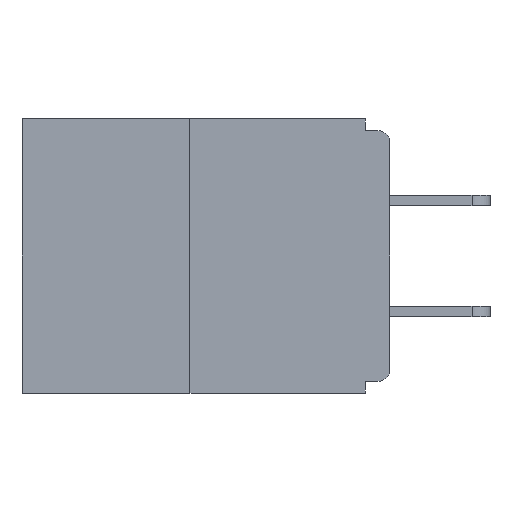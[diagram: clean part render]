
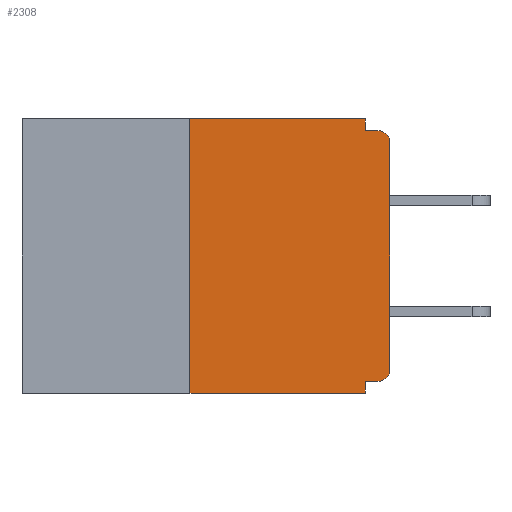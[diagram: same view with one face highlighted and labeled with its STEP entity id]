
A CAD part, left-side view. The second image highlights one B-rep face of the part: STEP entity #2308.
In plain terms, the highlighted planar face has unit normal (-1, 0, 0).
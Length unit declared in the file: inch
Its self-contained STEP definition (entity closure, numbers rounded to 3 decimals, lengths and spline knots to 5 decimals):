
#131 = CARTESIAN_POINT ( 'NONE',  ( 0., 0.25, -0.343 ) ) ;
#202 = CARTESIAN_POINT ( 'NONE',  ( 0., 0.46, 0. ) ) ;
#671 = DIRECTION ( 'NONE',  ( -1., 0., 0. ) ) ;
#1370 = VERTEX_POINT ( 'NONE', #13479 ) ;
#1559 = LINE ( 'NONE', #3961, #16559 ) ;
#1993 = DIRECTION ( 'NONE',  ( 0., 0., -1. ) ) ;
#2171 = DIRECTION ( 'NONE',  ( 0., -1., 0. ) ) ;
#2308 = ADVANCED_FACE ( 'NONE', ( #8596 ), #10376, .F. ) ;
#2383 = CARTESIAN_POINT ( 'NONE',  ( 0., 0.46, 0. ) ) ;
#2576 = VECTOR ( 'NONE', #9183, 39.37008 ) ;
#2650 = VERTEX_POINT ( 'NONE', #9824 ) ;
#3369 = EDGE_CURVE ( 'NONE', #5888, #11974, #8760, .T. ) ;
#3402 = CARTESIAN_POINT ( 'NONE',  ( 0., 0.25, 0. ) ) ;
#3457 = DIRECTION ( 'NONE',  ( -1., 0., 0. ) ) ;
#3500 = CARTESIAN_POINT ( 'NONE',  ( 0., 0.25, 0. ) ) ;
#3734 = VERTEX_POINT ( 'NONE', #15342 ) ;
#3848 = CARTESIAN_POINT ( 'NONE',  ( 0., 0., -0.03 ) ) ;
#3932 = EDGE_CURVE ( 'NONE', #2650, #1370, #5480, .T. ) ;
#3961 = CARTESIAN_POINT ( 'NONE',  ( 0., 0.46, -0.343 ) ) ;
#4158 = VECTOR ( 'NONE', #11463, 39.37008 ) ;
#4496 = VERTEX_POINT ( 'NONE', #15976 ) ;
#4717 = EDGE_CURVE ( 'NONE', #5970, #9330, #13332, .T. ) ;
#4718 = EDGE_CURVE ( 'NONE', #13329, #4496, #1559, .T. ) ;
#5480 = LINE ( 'NONE', #13097, #6284 ) ;
#5781 = AXIS2_PLACEMENT_3D ( 'NONE', #202, #12934, #7872 ) ;
#5888 = VERTEX_POINT ( 'NONE', #15579 ) ;
#5970 = VERTEX_POINT ( 'NONE', #11804 ) ;
#6000 = AXIS2_PLACEMENT_3D ( 'NONE', #8614, #671, #7072 ) ;
#6284 = VECTOR ( 'NONE', #15729, 39.37008 ) ;
#6303 = VECTOR ( 'NONE', #2171, 39.37008 ) ;
#6318 = AXIS2_PLACEMENT_3D ( 'NONE', #9764, #3457, #13645 ) ;
#6791 = DIRECTION ( 'NONE',  ( 0., 0., 1. ) ) ;
#7072 = DIRECTION ( 'NONE',  ( 0., 0., -1. ) ) ;
#7277 = CARTESIAN_POINT ( 'NONE',  ( 0., 0.031, 0. ) ) ;
#7509 = ORIENTED_EDGE ( 'NONE', *, *, #15427, .T. ) ;
#7675 = EDGE_LOOP ( 'NONE', ( #12702, #15462, #13352, #12269, #12485, #9810, #16734, #7509, #9203, #15698 ) ) ;
#7757 = LINE ( 'NONE', #3500, #10358 ) ;
#7872 = DIRECTION ( 'NONE',  ( 0., 0., -1. ) ) ;
#7903 = DIRECTION ( 'NONE',  ( 0., -1., 0. ) ) ;
#8468 = CIRCLE ( 'NONE', #6318, 0.015 ) ;
#8596 = FACE_OUTER_BOUND ( 'NONE', #7675, .T. ) ;
#8614 = CARTESIAN_POINT ( 'NONE',  ( 0., 0.015, -0.03 ) ) ;
#8716 = LINE ( 'NONE', #7277, #8897 ) ;
#8760 = LINE ( 'NONE', #16490, #6303 ) ;
#8884 = CIRCLE ( 'NONE', #6000, 0.015 ) ;
#8897 = VECTOR ( 'NONE', #1993, 39.37008 ) ;
#9183 = DIRECTION ( 'NONE',  ( 0., 0., 1. ) ) ;
#9203 = ORIENTED_EDGE ( 'NONE', *, *, #3369, .F. ) ;
#9330 = VERTEX_POINT ( 'NONE', #3848 ) ;
#9764 = CARTESIAN_POINT ( 'NONE',  ( 0., 0.015, -0.313 ) ) ;
#9810 = ORIENTED_EDGE ( 'NONE', *, *, #15857, .T. ) ;
#9824 = CARTESIAN_POINT ( 'NONE',  ( 0., 0.015, -0.328 ) ) ;
#10210 = EDGE_CURVE ( 'NONE', #3734, #5888, #8716, .T. ) ;
#10221 = VERTEX_POINT ( 'NONE', #3402 ) ;
#10358 = VECTOR ( 'NONE', #6791, 39.37008 ) ;
#10376 = PLANE ( 'NONE',  #5781 ) ;
#10467 = CARTESIAN_POINT ( 'NONE',  ( 0., 0., 0. ) ) ;
#10588 = DIRECTION ( 'NONE',  ( 0., 0., -1. ) ) ;
#11463 = DIRECTION ( 'NONE',  ( 0., -1., 0. ) ) ;
#11500 = EDGE_CURVE ( 'NONE', #10221, #3734, #11876, .T. ) ;
#11804 = CARTESIAN_POINT ( 'NONE',  ( 0., 0., -0.313 ) ) ;
#11876 = LINE ( 'NONE', #2383, #4158 ) ;
#11974 = VERTEX_POINT ( 'NONE', #16473 ) ;
#12269 = ORIENTED_EDGE ( 'NONE', *, *, #12414, .F. ) ;
#12336 = EDGE_CURVE ( 'NONE', #13329, #10221, #7757, .T. ) ;
#12414 = EDGE_CURVE ( 'NONE', #1370, #4496, #16222, .T. ) ;
#12485 = ORIENTED_EDGE ( 'NONE', *, *, #3932, .F. ) ;
#12599 = VECTOR ( 'NONE', #10588, 39.37008 ) ;
#12702 = ORIENTED_EDGE ( 'NONE', *, *, #11500, .F. ) ;
#12934 = DIRECTION ( 'NONE',  ( 1., 0., 0. ) ) ;
#13097 = CARTESIAN_POINT ( 'NONE',  ( 0., 0., -0.328 ) ) ;
#13329 = VERTEX_POINT ( 'NONE', #131 ) ;
#13332 = LINE ( 'NONE', #10467, #2576 ) ;
#13352 = ORIENTED_EDGE ( 'NONE', *, *, #4718, .T. ) ;
#13479 = CARTESIAN_POINT ( 'NONE',  ( 0., 0.031, -0.328 ) ) ;
#13645 = DIRECTION ( 'NONE',  ( 0., 0., -1. ) ) ;
#14961 = CARTESIAN_POINT ( 'NONE',  ( 0., 0.031, -0.343 ) ) ;
#15342 = CARTESIAN_POINT ( 'NONE',  ( 0., 0.031, 0. ) ) ;
#15427 = EDGE_CURVE ( 'NONE', #9330, #11974, #8884, .T. ) ;
#15462 = ORIENTED_EDGE ( 'NONE', *, *, #12336, .F. ) ;
#15579 = CARTESIAN_POINT ( 'NONE',  ( 0., 0.031, -0.015 ) ) ;
#15698 = ORIENTED_EDGE ( 'NONE', *, *, #10210, .F. ) ;
#15729 = DIRECTION ( 'NONE',  ( 0., 1., 0. ) ) ;
#15857 = EDGE_CURVE ( 'NONE', #2650, #5970, #8468, .T. ) ;
#15976 = CARTESIAN_POINT ( 'NONE',  ( 0., 0.031, -0.343 ) ) ;
#16222 = LINE ( 'NONE', #14961, #12599 ) ;
#16473 = CARTESIAN_POINT ( 'NONE',  ( 0., 0.015, -0.015 ) ) ;
#16490 = CARTESIAN_POINT ( 'NONE',  ( 0., 0., -0.015 ) ) ;
#16559 = VECTOR ( 'NONE', #7903, 39.37008 ) ;
#16734 = ORIENTED_EDGE ( 'NONE', *, *, #4717, .T. ) ;
